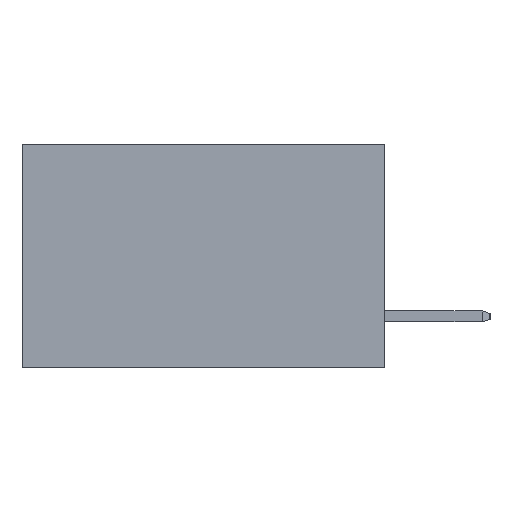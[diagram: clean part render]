
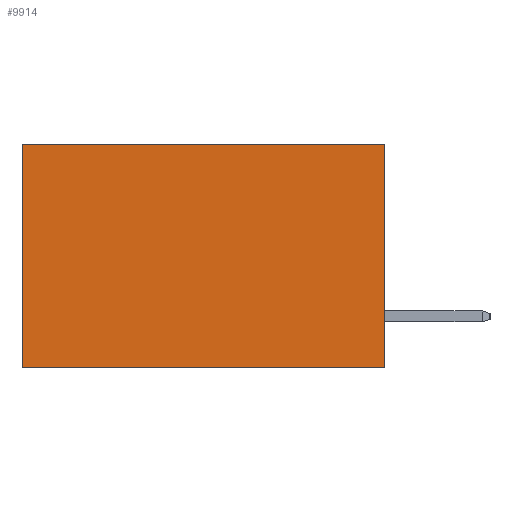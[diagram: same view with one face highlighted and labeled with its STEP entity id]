
A CAD part, left-side view. The second image highlights one B-rep face of the part: STEP entity #9914.
In plain terms, the highlighted planar face has unit normal (-1, 0, 0).
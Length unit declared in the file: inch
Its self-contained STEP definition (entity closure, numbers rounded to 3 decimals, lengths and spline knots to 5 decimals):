
#543 = EDGE_CURVE ( 'NONE', #2338, #11000, #9383, .T. ) ;
#719 = DIRECTION ( 'NONE',  ( 0., 0., -1. ) ) ;
#1047 = CARTESIAN_POINT ( 'NONE',  ( 0.2615, 0.6, -0.37 ) ) ;
#1062 = CARTESIAN_POINT ( 'NONE',  ( 0.2615, 0.6, 0. ) ) ;
#2169 = DIRECTION ( 'NONE',  ( 0., 1., 0. ) ) ;
#2228 = ORIENTED_EDGE ( 'NONE', *, *, #543, .F. ) ;
#2238 = CARTESIAN_POINT ( 'NONE',  ( 0.2615, 0.6, -0.37 ) ) ;
#2338 = VERTEX_POINT ( 'NONE', #8655 ) ;
#2612 = FACE_OUTER_BOUND ( 'NONE', #5008, .T. ) ;
#3158 = CARTESIAN_POINT ( 'NONE',  ( 0.2615, 0., 0. ) ) ;
#3760 = DIRECTION ( 'NONE',  ( 0., 0., -1. ) ) ;
#4045 = CARTESIAN_POINT ( 'NONE',  ( 0.2615, 0., -0.37 ) ) ;
#4540 = ORIENTED_EDGE ( 'NONE', *, *, #6395, .T. ) ;
#5008 = EDGE_LOOP ( 'NONE', ( #14597, #16095, #2228, #4540 ) ) ;
#5856 = VECTOR ( 'NONE', #12914, 39.37008 ) ;
#5978 = AXIS2_PLACEMENT_3D ( 'NONE', #16248, #8794, #719 ) ;
#5980 = EDGE_CURVE ( 'NONE', #11000, #7729, #13458, .T. ) ;
#6395 = EDGE_CURVE ( 'NONE', #2338, #14648, #12279, .T. ) ;
#7421 = PLANE ( 'NONE',  #5978 ) ;
#7729 = VERTEX_POINT ( 'NONE', #2238 ) ;
#8655 = CARTESIAN_POINT ( 'NONE',  ( 0.2615, 0., 0. ) ) ;
#8794 = DIRECTION ( 'NONE',  ( 1., 0., 0. ) ) ;
#9174 = VECTOR ( 'NONE', #3760, 39.37008 ) ;
#9383 = LINE ( 'NONE', #4045, #5856 ) ;
#9560 = LINE ( 'NONE', #1047, #9174 ) ;
#9914 = ADVANCED_FACE ( 'NONE', ( #2612 ), #7421, .F. ) ;
#10813 = CARTESIAN_POINT ( 'NONE',  ( 0.2615, 0., -0.37 ) ) ;
#11000 = VERTEX_POINT ( 'NONE', #10813 ) ;
#12279 = LINE ( 'NONE', #3158, #13064 ) ;
#12319 = DIRECTION ( 'NONE',  ( 0., 1., 0. ) ) ;
#12656 = CARTESIAN_POINT ( 'NONE',  ( 0.2615, 0., -0.37 ) ) ;
#12680 = VECTOR ( 'NONE', #2169, 39.37008 ) ;
#12914 = DIRECTION ( 'NONE',  ( 0., 0., -1. ) ) ;
#13064 = VECTOR ( 'NONE', #12319, 39.37008 ) ;
#13458 = LINE ( 'NONE', #12656, #12680 ) ;
#14597 = ORIENTED_EDGE ( 'NONE', *, *, #15945, .T. ) ;
#14648 = VERTEX_POINT ( 'NONE', #1062 ) ;
#15945 = EDGE_CURVE ( 'NONE', #14648, #7729, #9560, .T. ) ;
#16095 = ORIENTED_EDGE ( 'NONE', *, *, #5980, .F. ) ;
#16248 = CARTESIAN_POINT ( 'NONE',  ( 0.2615, 0., -0.37 ) ) ;
